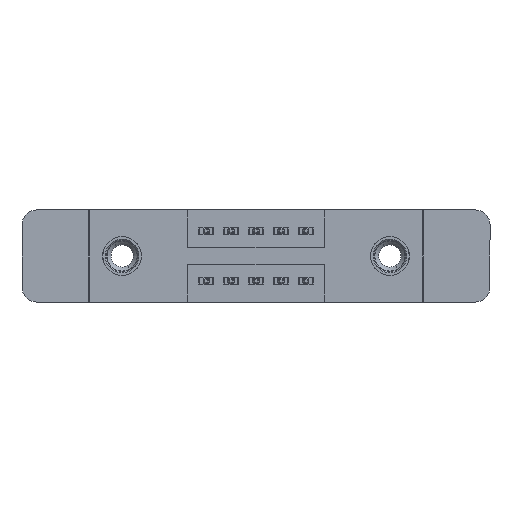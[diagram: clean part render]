
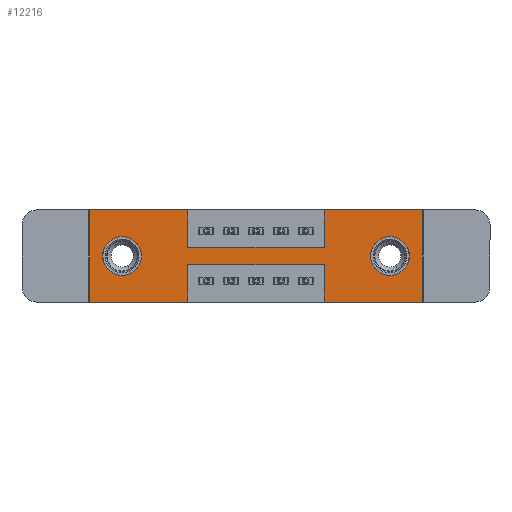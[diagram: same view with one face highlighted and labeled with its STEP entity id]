
A CAD part, front view. The second image highlights one B-rep face of the part: STEP entity #12216.
In plain terms, the highlighted planar face has unit normal (0, -1, 0).
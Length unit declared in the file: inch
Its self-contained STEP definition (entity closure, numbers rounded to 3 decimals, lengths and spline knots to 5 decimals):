
#71 = LINE ( 'NONE', #2920, #418 ) ;
#78 = EDGE_LOOP ( 'NONE', ( #5947, #560, #11278, #6687, #338, #7074, #3779, #12327, #4667, #5717, #1062, #11153 ) ) ;
#104 = VECTOR ( 'NONE', #1244, 39.37008 ) ;
#120 = CARTESIAN_POINT ( 'NONE',  ( 1.335, 0., -0.37 ) ) ;
#242 = VECTOR ( 'NONE', #4993, 39.37008 ) ;
#338 = ORIENTED_EDGE ( 'NONE', *, *, #3754, .F. ) ;
#399 = EDGE_CURVE ( 'NONE', #8590, #4471, #3264, .T. ) ;
#418 = VECTOR ( 'NONE', #10608, 39.37008 ) ;
#424 = DIRECTION ( 'NONE',  ( 0., 0., 1. ) ) ;
#449 = VECTOR ( 'NONE', #424, 39.37008 ) ;
#560 = ORIENTED_EDGE ( 'NONE', *, *, #9689, .F. ) ;
#600 = DIRECTION ( 'NONE',  ( 0., 0., -1. ) ) ;
#712 = ORIENTED_EDGE ( 'NONE', *, *, #4401, .T. ) ;
#791 = VERTEX_POINT ( 'NONE', #909 ) ;
#834 = DIRECTION ( 'NONE',  ( 0., -1., 0. ) ) ;
#909 = CARTESIAN_POINT ( 'NONE',  ( 0.13, 0., -0.263 ) ) ;
#1034 = VERTEX_POINT ( 'NONE', #3819 ) ;
#1062 = ORIENTED_EDGE ( 'NONE', *, *, #4096, .F. ) ;
#1206 = DIRECTION ( 'NONE',  ( 1., 0., 0. ) ) ;
#1244 = DIRECTION ( 'NONE',  ( 0., 0., -1. ) ) ;
#1371 = CIRCLE ( 'NONE', #3108, 0.078 ) ;
#1580 = CARTESIAN_POINT ( 'NONE',  ( 0.9425, 0., -0.37 ) ) ;
#1583 = CARTESIAN_POINT ( 'NONE',  ( 0.9425, 0., -0.37 ) ) ;
#1869 = DIRECTION ( 'NONE',  ( 0., 1., 0. ) ) ;
#1952 = VERTEX_POINT ( 'NONE', #8489 ) ;
#2041 = VERTEX_POINT ( 'NONE', #120 ) ;
#2138 = VERTEX_POINT ( 'NONE', #1583 ) ;
#2161 = LINE ( 'NONE', #12277, #4376 ) ;
#2305 = DIRECTION ( 'NONE',  ( 0., 0., -1. ) ) ;
#2365 = EDGE_CURVE ( 'NONE', #2041, #2138, #71, .T. ) ;
#2464 = DIRECTION ( 'NONE',  ( 0., 1., 0. ) ) ;
#2524 = LINE ( 'NONE', #1580, #4218 ) ;
#2670 = DIRECTION ( 'NONE',  ( 0., 1., 0. ) ) ;
#2773 = EDGE_CURVE ( 'NONE', #13903, #791, #12931, .T. ) ;
#2788 = CARTESIAN_POINT ( 'NONE',  ( 1.205, 0., -0.185 ) ) ;
#2849 = CARTESIAN_POINT ( 'NONE',  ( 0.3925, 0., 0. ) ) ;
#2920 = CARTESIAN_POINT ( 'NONE',  ( 0., 0., -0.37 ) ) ;
#2942 = CARTESIAN_POINT ( 'NONE',  ( 1.205, 0., -0.107 ) ) ;
#3108 = AXIS2_PLACEMENT_3D ( 'NONE', #2788, #2464, #600 ) ;
#3264 = CIRCLE ( 'NONE', #3751, 0.078 ) ;
#3401 = FACE_OUTER_BOUND ( 'NONE', #78, .T. ) ;
#3413 = LINE ( 'NONE', #5820, #449 ) ;
#3447 = DIRECTION ( 'NONE',  ( 0., 1., 0. ) ) ;
#3546 = LINE ( 'NONE', #4893, #242 ) ;
#3695 = DIRECTION ( 'NONE',  ( 0., 0., 1. ) ) ;
#3751 = AXIS2_PLACEMENT_3D ( 'NONE', #8945, #3447, #2305 ) ;
#3754 = EDGE_CURVE ( 'NONE', #10278, #2041, #2161, .T. ) ;
#3779 = ORIENTED_EDGE ( 'NONE', *, *, #11886, .F. ) ;
#3819 = CARTESIAN_POINT ( 'NONE',  ( 0.3925, 0., -0.22 ) ) ;
#4096 = EDGE_CURVE ( 'NONE', #9119, #9532, #8904, .T. ) ;
#4120 = LINE ( 'NONE', #13409, #12837 ) ;
#4218 = VECTOR ( 'NONE', #3695, 39.37008 ) ;
#4376 = VECTOR ( 'NONE', #6840, 39.37008 ) ;
#4401 = EDGE_CURVE ( 'NONE', #4471, #8590, #1371, .T. ) ;
#4471 = VERTEX_POINT ( 'NONE', #2942 ) ;
#4654 = CARTESIAN_POINT ( 'NONE',  ( 0.3925, 0., -0.15 ) ) ;
#4667 = ORIENTED_EDGE ( 'NONE', *, *, #6988, .F. ) ;
#4765 = CARTESIAN_POINT ( 'NONE',  ( 0., 0., 0. ) ) ;
#4893 = CARTESIAN_POINT ( 'NONE',  ( 0., 0., 0. ) ) ;
#4993 = DIRECTION ( 'NONE',  ( 1., 0., 0. ) ) ;
#5210 = CARTESIAN_POINT ( 'NONE',  ( 0.13, 0., -0.185 ) ) ;
#5308 = AXIS2_PLACEMENT_3D ( 'NONE', #5210, #1869, #10619 ) ;
#5337 = EDGE_CURVE ( 'NONE', #1034, #8244, #11604, .T. ) ;
#5383 = CIRCLE ( 'NONE', #5308, 0.078 ) ;
#5561 = VERTEX_POINT ( 'NONE', #2849 ) ;
#5688 = CARTESIAN_POINT ( 'NONE',  ( 0.3925, 0., -0.37 ) ) ;
#5717 = ORIENTED_EDGE ( 'NONE', *, *, #6477, .F. ) ;
#5820 = CARTESIAN_POINT ( 'NONE',  ( 0.9425, 0., 0. ) ) ;
#5947 = ORIENTED_EDGE ( 'NONE', *, *, #5337, .F. ) ;
#6390 = PLANE ( 'NONE',  #13457 ) ;
#6445 = LINE ( 'NONE', #8629, #8331 ) ;
#6477 = EDGE_CURVE ( 'NONE', #9532, #5561, #3546, .T. ) ;
#6687 = ORIENTED_EDGE ( 'NONE', *, *, #2365, .F. ) ;
#6717 = VERTEX_POINT ( 'NONE', #8126 ) ;
#6753 = CARTESIAN_POINT ( 'NONE',  ( 0.13, 0., -0.107 ) ) ;
#6840 = DIRECTION ( 'NONE',  ( 0., 0., -1. ) ) ;
#6988 = EDGE_CURVE ( 'NONE', #5561, #6717, #10375, .T. ) ;
#6990 = AXIS2_PLACEMENT_3D ( 'NONE', #12397, #2670, #8017 ) ;
#7074 = ORIENTED_EDGE ( 'NONE', *, *, #12711, .F. ) ;
#7223 = CARTESIAN_POINT ( 'NONE',  ( 0.9425, 0., 0. ) ) ;
#7383 = CARTESIAN_POINT ( 'NONE',  ( 0., 0., -0.37 ) ) ;
#7444 = VECTOR ( 'NONE', #8587, 39.37008 ) ;
#7615 = EDGE_CURVE ( 'NONE', #791, #13903, #5383, .T. ) ;
#7831 = CARTESIAN_POINT ( 'NONE',  ( 0.9425, 0., -0.22 ) ) ;
#7892 = DIRECTION ( 'NONE',  ( 1., 0., 0. ) ) ;
#8006 = FACE_BOUND ( 'NONE', #13110, .T. ) ;
#8017 = DIRECTION ( 'NONE',  ( 0., 0., 1. ) ) ;
#8126 = CARTESIAN_POINT ( 'NONE',  ( 0.3925, 0., -0.15 ) ) ;
#8244 = VERTEX_POINT ( 'NONE', #10795 ) ;
#8331 = VECTOR ( 'NONE', #1206, 39.37008 ) ;
#8423 = CARTESIAN_POINT ( 'NONE',  ( 1.335, 0., 0. ) ) ;
#8489 = CARTESIAN_POINT ( 'NONE',  ( 0.9425, 0., -0.15 ) ) ;
#8587 = DIRECTION ( 'NONE',  ( 0., 0., -1. ) ) ;
#8590 = VERTEX_POINT ( 'NONE', #11684 ) ;
#8629 = CARTESIAN_POINT ( 'NONE',  ( 0., 0., 0. ) ) ;
#8864 = EDGE_CURVE ( 'NONE', #8244, #9119, #14189, .T. ) ;
#8904 = LINE ( 'NONE', #4765, #10626 ) ;
#8945 = CARTESIAN_POINT ( 'NONE',  ( 1.205, 0., -0.185 ) ) ;
#9119 = VERTEX_POINT ( 'NONE', #13794 ) ;
#9156 = DIRECTION ( 'NONE',  ( -1., 0., 0. ) ) ;
#9181 = VERTEX_POINT ( 'NONE', #7223 ) ;
#9532 = VERTEX_POINT ( 'NONE', #9875 ) ;
#9616 = ORIENTED_EDGE ( 'NONE', *, *, #2773, .T. ) ;
#9689 = EDGE_CURVE ( 'NONE', #11796, #1034, #4120, .T. ) ;
#9875 = CARTESIAN_POINT ( 'NONE',  ( 0., 0., 0. ) ) ;
#10012 = ORIENTED_EDGE ( 'NONE', *, *, #7615, .T. ) ;
#10278 = VERTEX_POINT ( 'NONE', #8423 ) ;
#10317 = VECTOR ( 'NONE', #13088, 39.37008 ) ;
#10375 = LINE ( 'NONE', #11865, #7444 ) ;
#10608 = DIRECTION ( 'NONE',  ( -1., 0., 0. ) ) ;
#10619 = DIRECTION ( 'NONE',  ( 0., 0., 1. ) ) ;
#10626 = VECTOR ( 'NONE', #12389, 39.37008 ) ;
#10729 = LINE ( 'NONE', #4654, #11245 ) ;
#10787 = DIRECTION ( 'NONE',  ( 0., 0., -1. ) ) ;
#10795 = CARTESIAN_POINT ( 'NONE',  ( 0.3925, 0., -0.37 ) ) ;
#10999 = ORIENTED_EDGE ( 'NONE', *, *, #399, .T. ) ;
#11153 = ORIENTED_EDGE ( 'NONE', *, *, #8864, .F. ) ;
#11245 = VECTOR ( 'NONE', #7892, 39.37008 ) ;
#11278 = ORIENTED_EDGE ( 'NONE', *, *, #12969, .F. ) ;
#11604 = LINE ( 'NONE', #5688, #104 ) ;
#11684 = CARTESIAN_POINT ( 'NONE',  ( 1.205, 0., -0.263 ) ) ;
#11796 = VERTEX_POINT ( 'NONE', #7831 ) ;
#11865 = CARTESIAN_POINT ( 'NONE',  ( 0.3925, 0., 0. ) ) ;
#11886 = EDGE_CURVE ( 'NONE', #1952, #9181, #3413, .T. ) ;
#12216 = ADVANCED_FACE ( 'NONE', ( #12434, #8006, #3401 ), #6390, .T. ) ;
#12277 = CARTESIAN_POINT ( 'NONE',  ( 1.335, 0., 0. ) ) ;
#12327 = ORIENTED_EDGE ( 'NONE', *, *, #12910, .F. ) ;
#12389 = DIRECTION ( 'NONE',  ( 0., 0., 1. ) ) ;
#12397 = CARTESIAN_POINT ( 'NONE',  ( 0.13, 0., -0.185 ) ) ;
#12434 = FACE_BOUND ( 'NONE', #13397, .T. ) ;
#12711 = EDGE_CURVE ( 'NONE', #9181, #10278, #6445, .T. ) ;
#12837 = VECTOR ( 'NONE', #9156, 39.37008 ) ;
#12910 = EDGE_CURVE ( 'NONE', #6717, #1952, #10729, .T. ) ;
#12931 = CIRCLE ( 'NONE', #6990, 0.078 ) ;
#12969 = EDGE_CURVE ( 'NONE', #2138, #11796, #2524, .T. ) ;
#13088 = DIRECTION ( 'NONE',  ( -1., 0., 0. ) ) ;
#13110 = EDGE_LOOP ( 'NONE', ( #9616, #10012 ) ) ;
#13231 = CARTESIAN_POINT ( 'NONE',  ( 0., 0., -0.37 ) ) ;
#13397 = EDGE_LOOP ( 'NONE', ( #712, #10999 ) ) ;
#13409 = CARTESIAN_POINT ( 'NONE',  ( 0.3925, 0., -0.22 ) ) ;
#13457 = AXIS2_PLACEMENT_3D ( 'NONE', #7383, #834, #10787 ) ;
#13794 = CARTESIAN_POINT ( 'NONE',  ( 0., 0., -0.37 ) ) ;
#13903 = VERTEX_POINT ( 'NONE', #6753 ) ;
#14189 = LINE ( 'NONE', #13231, #10317 ) ;
